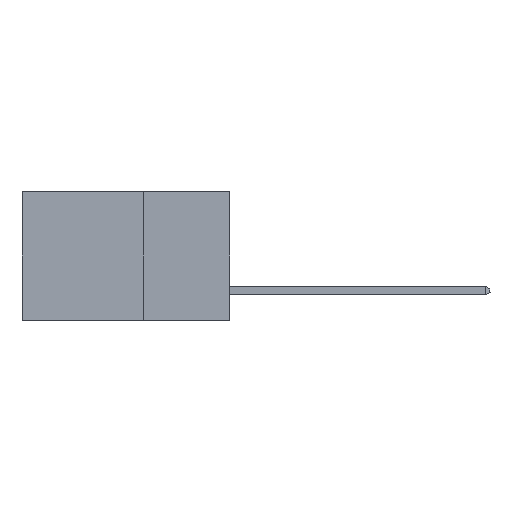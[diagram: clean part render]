
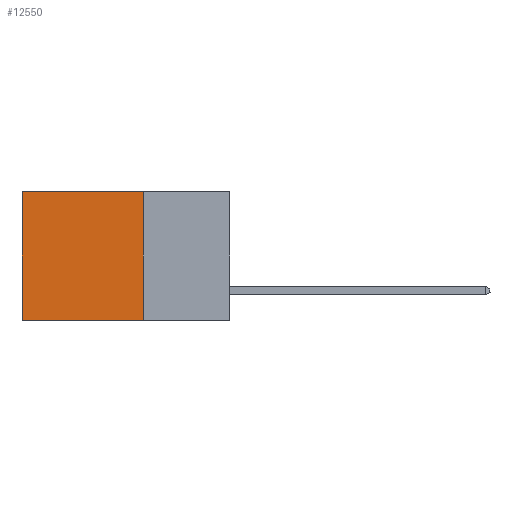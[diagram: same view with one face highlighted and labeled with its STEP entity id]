
A CAD part, left-side view. The second image highlights one B-rep face of the part: STEP entity #12550.
In plain terms, the highlighted planar face has unit normal (-1, 0, 0).
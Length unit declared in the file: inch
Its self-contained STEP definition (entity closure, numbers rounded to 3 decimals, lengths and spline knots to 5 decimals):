
#200 = VECTOR ( 'NONE', #9378, 39.37008 ) ;
#572 = LINE ( 'NONE', #15456, #7321 ) ;
#1795 = VERTEX_POINT ( 'NONE', #3586 ) ;
#2545 = FACE_OUTER_BOUND ( 'NONE', #3619, .T. ) ;
#3014 = CARTESIAN_POINT ( 'NONE',  ( 0.298, 0.6, 0. ) ) ;
#3586 = CARTESIAN_POINT ( 'NONE',  ( 0.298, 0.6, 0. ) ) ;
#3619 = EDGE_LOOP ( 'NONE', ( #22149, #6941, #20543, #23045 ) ) ;
#3968 = EDGE_CURVE ( 'NONE', #1795, #20154, #6842, .T. ) ;
#4687 = VERTEX_POINT ( 'NONE', #17966 ) ;
#5153 = DIRECTION ( 'NONE',  ( 0., 0., -1. ) ) ;
#5398 = CARTESIAN_POINT ( 'NONE',  ( 0.298, 0.25, 0. ) ) ;
#6842 = LINE ( 'NONE', #3014, #11739 ) ;
#6941 = ORIENTED_EDGE ( 'NONE', *, *, #11992, .F. ) ;
#6963 = VERTEX_POINT ( 'NONE', #15812 ) ;
#7321 = VECTOR ( 'NONE', #5153, 39.37008 ) ;
#7384 = DIRECTION ( 'NONE',  ( 0., 1., 0. ) ) ;
#9378 = DIRECTION ( 'NONE',  ( 0., 1., 0. ) ) ;
#11739 = VECTOR ( 'NONE', #13331, 39.37008 ) ;
#11880 = CARTESIAN_POINT ( 'NONE',  ( 0.298, 0.25, 0. ) ) ;
#11992 = EDGE_CURVE ( 'NONE', #4687, #20154, #25617, .T. ) ;
#12550 = ADVANCED_FACE ( 'NONE', ( #2545 ), #26297, .F. ) ;
#13331 = DIRECTION ( 'NONE',  ( 0., 0., -1. ) ) ;
#13561 = EDGE_CURVE ( 'NONE', #6963, #1795, #15109, .T. ) ;
#14644 = DIRECTION ( 'NONE',  ( 0., 0., -1. ) ) ;
#15109 = LINE ( 'NONE', #5398, #200 ) ;
#15456 = CARTESIAN_POINT ( 'NONE',  ( 0.298, 0.25, 0. ) ) ;
#15812 = CARTESIAN_POINT ( 'NONE',  ( 0.298, 0.25, 0. ) ) ;
#17966 = CARTESIAN_POINT ( 'NONE',  ( 0.298, 0.25, -0.37 ) ) ;
#19051 = EDGE_CURVE ( 'NONE', #6963, #4687, #572, .T. ) ;
#20154 = VERTEX_POINT ( 'NONE', #21147 ) ;
#20452 = VECTOR ( 'NONE', #7384, 39.37008 ) ;
#20543 = ORIENTED_EDGE ( 'NONE', *, *, #19051, .F. ) ;
#21147 = CARTESIAN_POINT ( 'NONE',  ( 0.298, 0.6, -0.37 ) ) ;
#22149 = ORIENTED_EDGE ( 'NONE', *, *, #3968, .T. ) ;
#23045 = ORIENTED_EDGE ( 'NONE', *, *, #13561, .T. ) ;
#24938 = AXIS2_PLACEMENT_3D ( 'NONE', #11880, #26394, #14644 ) ;
#25617 = LINE ( 'NONE', #25987, #20452 ) ;
#25987 = CARTESIAN_POINT ( 'NONE',  ( 0.298, 0.25, -0.37 ) ) ;
#26297 = PLANE ( 'NONE',  #24938 ) ;
#26394 = DIRECTION ( 'NONE',  ( 1., 0., 0. ) ) ;
